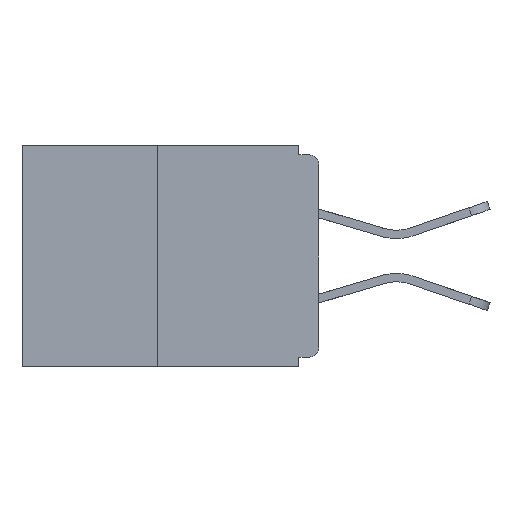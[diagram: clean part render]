
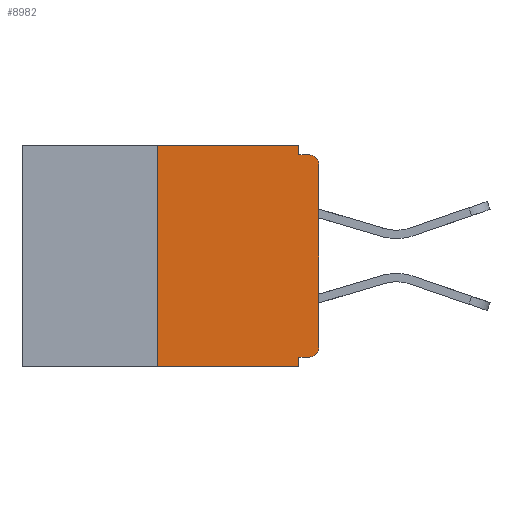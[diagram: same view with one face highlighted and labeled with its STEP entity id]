
A CAD part, left-side view. The second image highlights one B-rep face of the part: STEP entity #8982.
In plain terms, the highlighted planar face has unit normal (-1, 0, 0).
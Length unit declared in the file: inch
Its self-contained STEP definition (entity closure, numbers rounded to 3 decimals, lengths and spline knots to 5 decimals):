
#451 = CARTESIAN_POINT ( 'NONE',  ( 0., 0., 0. ) ) ;
#634 = VERTEX_POINT ( 'NONE', #21115 ) ;
#825 = VECTOR ( 'NONE', #12614, 39.37008 ) ;
#1113 = CARTESIAN_POINT ( 'NONE',  ( 0., 0., -0.015 ) ) ;
#1658 = VERTEX_POINT ( 'NONE', #6845 ) ;
#2285 = DIRECTION ( 'NONE',  ( 0., 0., 1. ) ) ;
#2322 = LINE ( 'NONE', #15808, #4693 ) ;
#2357 = CARTESIAN_POINT ( 'NONE',  ( 0., 0.031, 0. ) ) ;
#3257 = DIRECTION ( 'NONE',  ( 0., 0., -1. ) ) ;
#3605 = CARTESIAN_POINT ( 'NONE',  ( 0., 0.031, -0.328 ) ) ;
#4435 = VECTOR ( 'NONE', #8291, 39.37008 ) ;
#4693 = VECTOR ( 'NONE', #4879, 39.37008 ) ;
#4797 = VERTEX_POINT ( 'NONE', #3605 ) ;
#4879 = DIRECTION ( 'NONE',  ( 0., 0., -1. ) ) ;
#4982 = EDGE_CURVE ( 'NONE', #14209, #22211, #22952, .T. ) ;
#5181 = PLANE ( 'NONE',  #8755 ) ;
#5251 = EDGE_CURVE ( 'NONE', #1658, #15854, #24238, .T. ) ;
#5604 = CARTESIAN_POINT ( 'NONE',  ( 0., 0.015, -0.313 ) ) ;
#5792 = VECTOR ( 'NONE', #10678, 39.37008 ) ;
#5861 = ORIENTED_EDGE ( 'NONE', *, *, #16909, .T. ) ;
#6085 = CIRCLE ( 'NONE', #11675, 0.015 ) ;
#6091 = FACE_OUTER_BOUND ( 'NONE', #12379, .T. ) ;
#6761 = CIRCLE ( 'NONE', #22775, 0.015 ) ;
#6845 = CARTESIAN_POINT ( 'NONE',  ( 0., 0.25, 0. ) ) ;
#7132 = ORIENTED_EDGE ( 'NONE', *, *, #8348, .T. ) ;
#7958 = DIRECTION ( 'NONE',  ( -1., 0., 0. ) ) ;
#8291 = DIRECTION ( 'NONE',  ( 0., 1., 0. ) ) ;
#8348 = EDGE_CURVE ( 'NONE', #25225, #21961, #6085, .T. ) ;
#8493 = ORIENTED_EDGE ( 'NONE', *, *, #5251, .F. ) ;
#8755 = AXIS2_PLACEMENT_3D ( 'NONE', #26790, #20385, #13859 ) ;
#8982 = ADVANCED_FACE ( 'NONE', ( #6091 ), #5181, .F. ) ;
#9393 = VECTOR ( 'NONE', #2285, 39.37008 ) ;
#9500 = CARTESIAN_POINT ( 'NONE',  ( 0., 0.031, -0.343 ) ) ;
#10148 = ORIENTED_EDGE ( 'NONE', *, *, #25774, .T. ) ;
#10428 = VERTEX_POINT ( 'NONE', #11586 ) ;
#10628 = CARTESIAN_POINT ( 'NONE',  ( 0., 0.46, -0.343 ) ) ;
#10678 = DIRECTION ( 'NONE',  ( 0., 0., -1. ) ) ;
#10768 = CARTESIAN_POINT ( 'NONE',  ( 0., 0.031, -0.343 ) ) ;
#11586 = CARTESIAN_POINT ( 'NONE',  ( 0., 0., -0.03 ) ) ;
#11675 = AXIS2_PLACEMENT_3D ( 'NONE', #5604, #7958, #16630 ) ;
#11761 = EDGE_CURVE ( 'NONE', #4797, #22211, #18006, .T. ) ;
#12379 = EDGE_LOOP ( 'NONE', ( #8493, #16744, #19817, #17515, #24582, #7132, #10148, #5861, #17299, #14336 ) ) ;
#12496 = VECTOR ( 'NONE', #27451, 39.37008 ) ;
#12604 = VERTEX_POINT ( 'NONE', #18512 ) ;
#12614 = DIRECTION ( 'NONE',  ( 0., -1., 0. ) ) ;
#12681 = CARTESIAN_POINT ( 'NONE',  ( 0., 0.25, 0. ) ) ;
#13006 = DIRECTION ( 'NONE',  ( 0., -1., 0. ) ) ;
#13520 = CARTESIAN_POINT ( 'NONE',  ( 0., 0.015, -0.328 ) ) ;
#13736 = LINE ( 'NONE', #1113, #16785 ) ;
#13859 = DIRECTION ( 'NONE',  ( 0., 0., -1. ) ) ;
#13972 = LINE ( 'NONE', #18944, #4435 ) ;
#14209 = VERTEX_POINT ( 'NONE', #15995 ) ;
#14336 = ORIENTED_EDGE ( 'NONE', *, *, #17357, .F. ) ;
#15085 = CARTESIAN_POINT ( 'NONE',  ( 0., 0., -0.313 ) ) ;
#15299 = EDGE_CURVE ( 'NONE', #12604, #634, #13736, .T. ) ;
#15808 = CARTESIAN_POINT ( 'NONE',  ( 0., 0.031, 0. ) ) ;
#15854 = VERTEX_POINT ( 'NONE', #2357 ) ;
#15995 = CARTESIAN_POINT ( 'NONE',  ( 0., 0.25, -0.343 ) ) ;
#16326 = DIRECTION ( 'NONE',  ( 0., -1., 0. ) ) ;
#16630 = DIRECTION ( 'NONE',  ( 0., 0., -1. ) ) ;
#16744 = ORIENTED_EDGE ( 'NONE', *, *, #26393, .F. ) ;
#16785 = VECTOR ( 'NONE', #16326, 39.37008 ) ;
#16909 = EDGE_CURVE ( 'NONE', #10428, #634, #6761, .T. ) ;
#17299 = ORIENTED_EDGE ( 'NONE', *, *, #15299, .F. ) ;
#17357 = EDGE_CURVE ( 'NONE', #15854, #12604, #2322, .T. ) ;
#17515 = ORIENTED_EDGE ( 'NONE', *, *, #11761, .F. ) ;
#18006 = LINE ( 'NONE', #10768, #5792 ) ;
#18512 = CARTESIAN_POINT ( 'NONE',  ( 0., 0.031, -0.015 ) ) ;
#18944 = CARTESIAN_POINT ( 'NONE',  ( 0., 0., -0.328 ) ) ;
#19817 = ORIENTED_EDGE ( 'NONE', *, *, #4982, .T. ) ;
#19969 = LINE ( 'NONE', #451, #9393 ) ;
#20385 = DIRECTION ( 'NONE',  ( 1., 0., 0. ) ) ;
#21115 = CARTESIAN_POINT ( 'NONE',  ( 0., 0.015, -0.015 ) ) ;
#21961 = VERTEX_POINT ( 'NONE', #15085 ) ;
#22211 = VERTEX_POINT ( 'NONE', #9500 ) ;
#22744 = CARTESIAN_POINT ( 'NONE',  ( 0., 0.015, -0.03 ) ) ;
#22775 = AXIS2_PLACEMENT_3D ( 'NONE', #22744, #22923, #3257 ) ;
#22923 = DIRECTION ( 'NONE',  ( -1., 0., 0. ) ) ;
#22952 = LINE ( 'NONE', #10628, #24262 ) ;
#24052 = EDGE_CURVE ( 'NONE', #25225, #4797, #13972, .T. ) ;
#24238 = LINE ( 'NONE', #25557, #825 ) ;
#24262 = VECTOR ( 'NONE', #13006, 39.37008 ) ;
#24582 = ORIENTED_EDGE ( 'NONE', *, *, #24052, .F. ) ;
#25225 = VERTEX_POINT ( 'NONE', #13520 ) ;
#25557 = CARTESIAN_POINT ( 'NONE',  ( 0., 0.46, 0. ) ) ;
#25774 = EDGE_CURVE ( 'NONE', #21961, #10428, #19969, .T. ) ;
#26393 = EDGE_CURVE ( 'NONE', #14209, #1658, #28061, .T. ) ;
#26790 = CARTESIAN_POINT ( 'NONE',  ( 0., 0.46, 0. ) ) ;
#27451 = DIRECTION ( 'NONE',  ( 0., 0., 1. ) ) ;
#28061 = LINE ( 'NONE', #12681, #12496 ) ;
